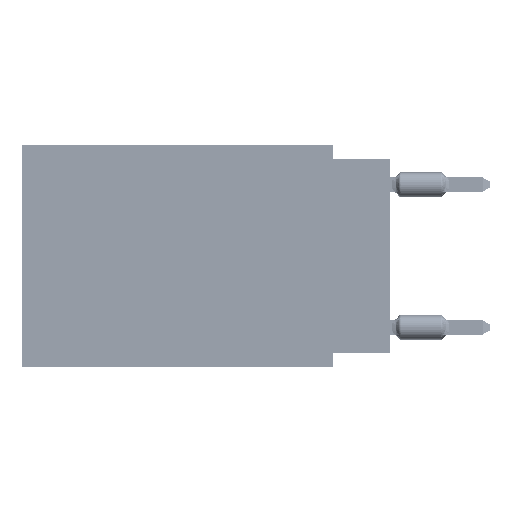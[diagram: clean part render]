
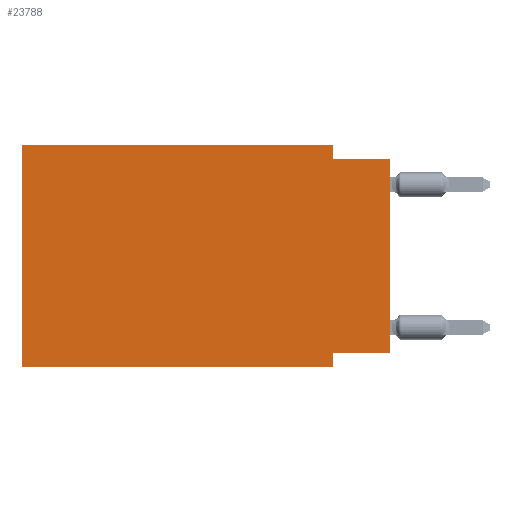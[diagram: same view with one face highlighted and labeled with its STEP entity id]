
A CAD part, left-side view. The second image highlights one B-rep face of the part: STEP entity #23788.
In plain terms, the highlighted planar face has unit normal (-1, 0, 0).
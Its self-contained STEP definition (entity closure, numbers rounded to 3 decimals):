
#118 = VERTEX_POINT ( 'NONE', #76399 ) ;
#4557 = AXIS2_PLACEMENT_3D ( 'NONE', #77423, #47679, #71552 ) ;
#4597 = DIRECTION ( 'NONE',  ( 0., 0., 1. ) ) ;
#6203 = VECTOR ( 'NONE', #16684, 1000. ) ;
#6924 = CARTESIAN_POINT ( 'NONE',  ( 0., 16.383, 0. ) ) ;
#8545 = LINE ( 'NONE', #44983, #51309 ) ;
#9757 = EDGE_LOOP ( 'NONE', ( #19951, #19479, #49032, #68429, #62243, #56313, #14173, #52722 ) ) ;
#13921 = VECTOR ( 'NONE', #28177, 1000. ) ;
#14173 = ORIENTED_EDGE ( 'NONE', *, *, #32550, .F. ) ;
#14200 = EDGE_CURVE ( 'NONE', #118, #65810, #8545, .T. ) ;
#15560 = CARTESIAN_POINT ( 'NONE',  ( 0., 2.54, -9.906 ) ) ;
#15687 = CARTESIAN_POINT ( 'NONE',  ( 0., 16.383, 0. ) ) ;
#16469 = VERTEX_POINT ( 'NONE', #70759 ) ;
#16684 = DIRECTION ( 'NONE',  ( 0., -1., 0. ) ) ;
#18129 = CARTESIAN_POINT ( 'NONE',  ( 0., 0., -0.635 ) ) ;
#18802 = VECTOR ( 'NONE', #75969, 1000. ) ;
#19479 = ORIENTED_EDGE ( 'NONE', *, *, #54832, .F. ) ;
#19951 = ORIENTED_EDGE ( 'NONE', *, *, #14200, .T. ) ;
#20663 = LINE ( 'NONE', #61789, #32599 ) ;
#21601 = VERTEX_POINT ( 'NONE', #30217 ) ;
#21807 = CARTESIAN_POINT ( 'NONE',  ( 0., 16.383, -9.906 ) ) ;
#21890 = VERTEX_POINT ( 'NONE', #52470 ) ;
#23182 = LINE ( 'NONE', #52954, #54219 ) ;
#23788 = ADVANCED_FACE ( 'NONE', ( #30048 ), #53547, .F. ) ;
#24945 = LINE ( 'NONE', #6924, #74817 ) ;
#25990 = CARTESIAN_POINT ( 'NONE',  ( 0., 2.54, 0. ) ) ;
#28177 = DIRECTION ( 'NONE',  ( 0., -1., 0. ) ) ;
#30048 = FACE_OUTER_BOUND ( 'NONE', #9757, .T. ) ;
#30217 = CARTESIAN_POINT ( 'NONE',  ( 0., 2.54, -9.906 ) ) ;
#31180 = VECTOR ( 'NONE', #39436, 1000. ) ;
#31595 = EDGE_CURVE ( 'NONE', #16469, #60698, #24945, .T. ) ;
#31740 = VERTEX_POINT ( 'NONE', #45280 ) ;
#31977 = DIRECTION ( 'NONE',  ( 0., -1., 0. ) ) ;
#32550 = EDGE_CURVE ( 'NONE', #58186, #21601, #64470, .T. ) ;
#32599 = VECTOR ( 'NONE', #61007, 1000. ) ;
#33028 = CARTESIAN_POINT ( 'NONE',  ( 0., 2.54, -9.271 ) ) ;
#36169 = EDGE_CURVE ( 'NONE', #21890, #16469, #40326, .T. ) ;
#39436 = DIRECTION ( 'NONE',  ( 0., 0., -1. ) ) ;
#39924 = CARTESIAN_POINT ( 'NONE',  ( 0., 0., -0.635 ) ) ;
#40326 = LINE ( 'NONE', #15687, #18802 ) ;
#44983 = CARTESIAN_POINT ( 'NONE',  ( 0., 0., 0. ) ) ;
#45280 = CARTESIAN_POINT ( 'NONE',  ( 0., 2.54, -0.635 ) ) ;
#47679 = DIRECTION ( 'NONE',  ( 1., 0., 0. ) ) ;
#48627 = DIRECTION ( 'NONE',  ( 0., 0., -1. ) ) ;
#49032 = ORIENTED_EDGE ( 'NONE', *, *, #57242, .F. ) ;
#51309 = VECTOR ( 'NONE', #4597, 1000. ) ;
#52470 = CARTESIAN_POINT ( 'NONE',  ( 0., 16.383, -9.906 ) ) ;
#52722 = ORIENTED_EDGE ( 'NONE', *, *, #67673, .F. ) ;
#52954 = CARTESIAN_POINT ( 'NONE',  ( 0., 2.54, 0. ) ) ;
#53547 = PLANE ( 'NONE',  #4557 ) ;
#54219 = VECTOR ( 'NONE', #48627, 1000. ) ;
#54295 = LINE ( 'NONE', #39924, #13921 ) ;
#54832 = EDGE_CURVE ( 'NONE', #31740, #65810, #54295, .T. ) ;
#56313 = ORIENTED_EDGE ( 'NONE', *, *, #66585, .T. ) ;
#57242 = EDGE_CURVE ( 'NONE', #60698, #31740, #23182, .T. ) ;
#58186 = VERTEX_POINT ( 'NONE', #33028 ) ;
#60698 = VERTEX_POINT ( 'NONE', #25990 ) ;
#61007 = DIRECTION ( 'NONE',  ( 0., 1., 0. ) ) ;
#61789 = CARTESIAN_POINT ( 'NONE',  ( 0., 0., -9.271 ) ) ;
#62243 = ORIENTED_EDGE ( 'NONE', *, *, #36169, .F. ) ;
#64470 = LINE ( 'NONE', #15560, #31180 ) ;
#65810 = VERTEX_POINT ( 'NONE', #18129 ) ;
#66585 = EDGE_CURVE ( 'NONE', #21890, #21601, #75450, .T. ) ;
#67673 = EDGE_CURVE ( 'NONE', #118, #58186, #20663, .T. ) ;
#68429 = ORIENTED_EDGE ( 'NONE', *, *, #31595, .F. ) ;
#70759 = CARTESIAN_POINT ( 'NONE',  ( 0., 16.383, 0. ) ) ;
#71552 = DIRECTION ( 'NONE',  ( 0., 0., -1. ) ) ;
#74817 = VECTOR ( 'NONE', #31977, 1000. ) ;
#75450 = LINE ( 'NONE', #21807, #6203 ) ;
#75969 = DIRECTION ( 'NONE',  ( 0., 0., 1. ) ) ;
#76399 = CARTESIAN_POINT ( 'NONE',  ( 0., 0., -9.271 ) ) ;
#77423 = CARTESIAN_POINT ( 'NONE',  ( 0., 16.383, 0. ) ) ;
